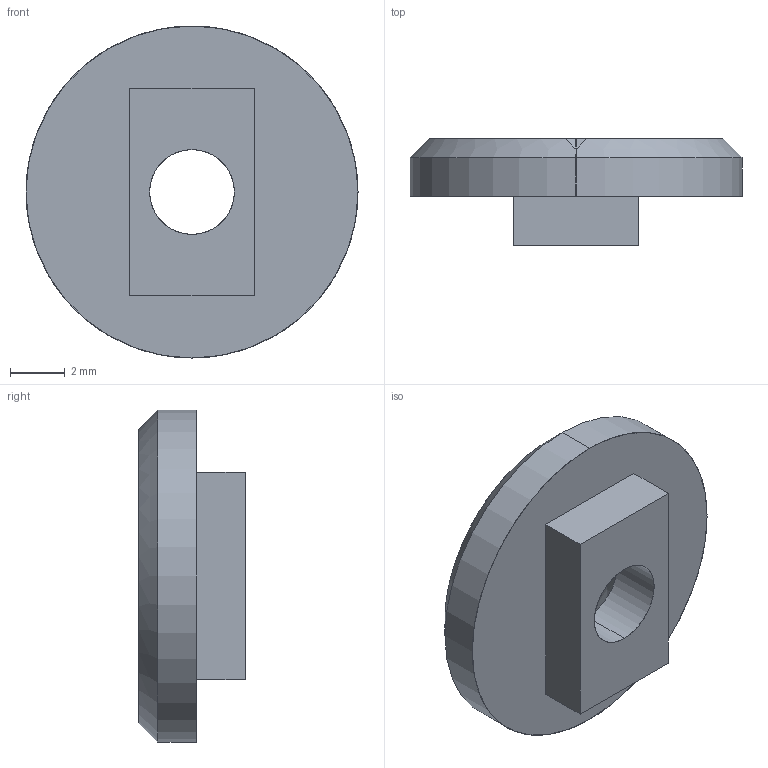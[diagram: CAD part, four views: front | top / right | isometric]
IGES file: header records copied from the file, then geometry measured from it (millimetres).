
Start section: SolidWorks IGES file using analytic representation for surfaces
Global section: file name: Lever_Cover.igs; native system: SolidWorks 2015; preprocessor: SolidWorks 2015; author: WarFairy; date: 150711.203100; units: millimetre
Bounding box: 12.17 x 3.91 x 12.17 mm (x, y, z)
Surface area: 359.1 mm2 (no closed solid volume)
Topology: 0 solids, 0 shells, 17 faces, 198 edges, 198 vertices
Faces by surface type: bspline 9, revolution 8
